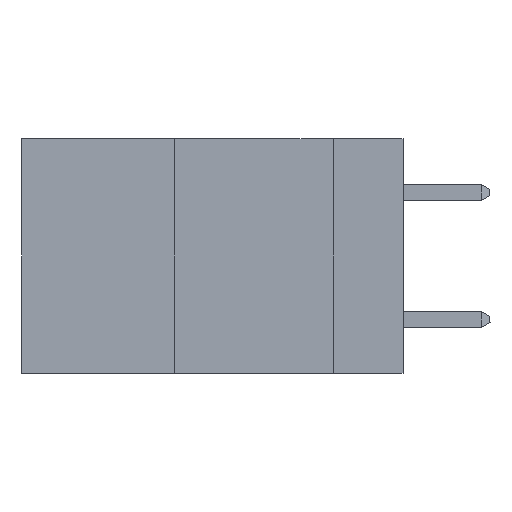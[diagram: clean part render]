
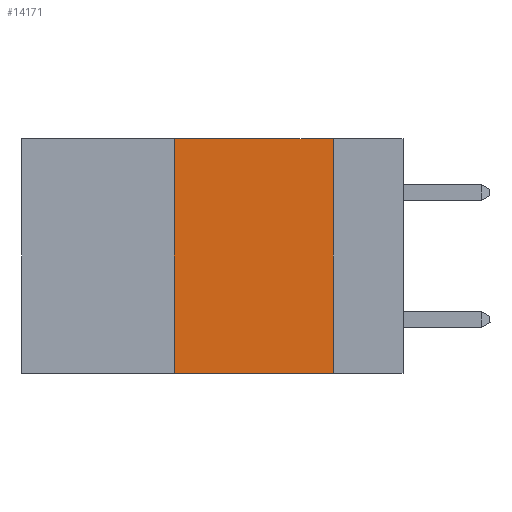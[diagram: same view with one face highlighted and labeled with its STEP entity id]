
A CAD part, left-side view. The second image highlights one B-rep face of the part: STEP entity #14171.
In plain terms, the highlighted planar face has unit normal (-1, 0, 0).
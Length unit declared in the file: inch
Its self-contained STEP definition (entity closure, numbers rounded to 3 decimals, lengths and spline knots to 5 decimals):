
#110 = VECTOR ( 'NONE', #4883, 39.37008 ) ;
#301 = LINE ( 'NONE', #7890, #12679 ) ;
#632 = ORIENTED_EDGE ( 'NONE', *, *, #5911, .F. ) ;
#789 = VECTOR ( 'NONE', #8062, 39.37008 ) ;
#800 = CARTESIAN_POINT ( 'NONE',  ( 0., 0.6, 0. ) ) ;
#1928 = CARTESIAN_POINT ( 'NONE',  ( 0., 0.36, 0. ) ) ;
#2799 = CARTESIAN_POINT ( 'NONE',  ( 0., 0.11, -0.37 ) ) ;
#2804 = EDGE_CURVE ( 'NONE', #10301, #14530, #301, .T. ) ;
#3089 = CARTESIAN_POINT ( 'NONE',  ( 0., 0.36, 0. ) ) ;
#3291 = EDGE_CURVE ( 'NONE', #10301, #12261, #15037, .T. ) ;
#3356 = EDGE_LOOP ( 'NONE', ( #15180, #632, #4089, #9325 ) ) ;
#4089 = ORIENTED_EDGE ( 'NONE', *, *, #3291, .F. ) ;
#4217 = DIRECTION ( 'NONE',  ( 0., 0., -1. ) ) ;
#4356 = FACE_OUTER_BOUND ( 'NONE', #3356, .T. ) ;
#4448 = LINE ( 'NONE', #800, #789 ) ;
#4883 = DIRECTION ( 'NONE',  ( 0., 0., -1. ) ) ;
#5391 = DIRECTION ( 'NONE',  ( 0., 0., 1. ) ) ;
#5911 = EDGE_CURVE ( 'NONE', #12261, #11238, #4448, .T. ) ;
#7890 = CARTESIAN_POINT ( 'NONE',  ( 0., 0.6, -0.37 ) ) ;
#8062 = DIRECTION ( 'NONE',  ( 0., -1., 0. ) ) ;
#8970 = PLANE ( 'NONE',  #12760 ) ;
#9184 = VECTOR ( 'NONE', #5391, 39.37008 ) ;
#9325 = ORIENTED_EDGE ( 'NONE', *, *, #2804, .T. ) ;
#10146 = CARTESIAN_POINT ( 'NONE',  ( 0., 0.6, 0. ) ) ;
#10301 = VERTEX_POINT ( 'NONE', #14980 ) ;
#11238 = VERTEX_POINT ( 'NONE', #11956 ) ;
#11341 = DIRECTION ( 'NONE',  ( 1., 0., 0. ) ) ;
#11956 = CARTESIAN_POINT ( 'NONE',  ( 0., 0.11, 0. ) ) ;
#12261 = VERTEX_POINT ( 'NONE', #1928 ) ;
#12570 = EDGE_CURVE ( 'NONE', #11238, #14530, #12856, .T. ) ;
#12611 = DIRECTION ( 'NONE',  ( 0., -1., 0. ) ) ;
#12679 = VECTOR ( 'NONE', #12611, 39.37008 ) ;
#12760 = AXIS2_PLACEMENT_3D ( 'NONE', #10146, #11341, #4217 ) ;
#12856 = LINE ( 'NONE', #13153, #110 ) ;
#13153 = CARTESIAN_POINT ( 'NONE',  ( 0., 0.11, 0. ) ) ;
#14171 = ADVANCED_FACE ( 'NONE', ( #4356 ), #8970, .F. ) ;
#14530 = VERTEX_POINT ( 'NONE', #2799 ) ;
#14980 = CARTESIAN_POINT ( 'NONE',  ( 0., 0.36, -0.37 ) ) ;
#15037 = LINE ( 'NONE', #3089, #9184 ) ;
#15180 = ORIENTED_EDGE ( 'NONE', *, *, #12570, .F. ) ;
